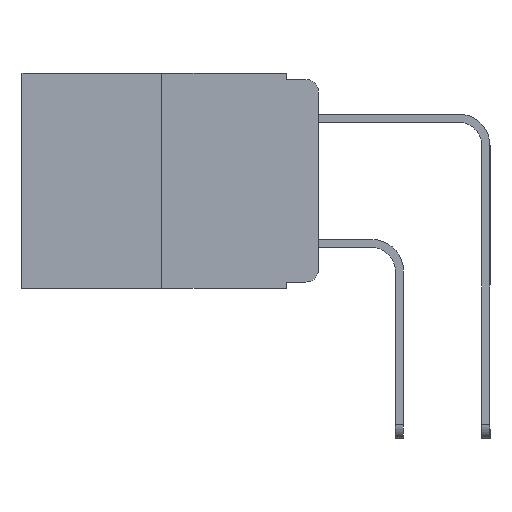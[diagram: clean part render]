
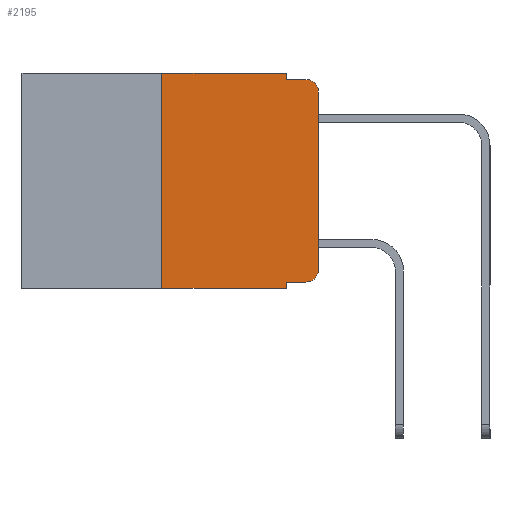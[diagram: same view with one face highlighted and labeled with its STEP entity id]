
A CAD part, left-side view. The second image highlights one B-rep face of the part: STEP entity #2195.
In plain terms, the highlighted planar face has unit normal (-1, 0, 0).
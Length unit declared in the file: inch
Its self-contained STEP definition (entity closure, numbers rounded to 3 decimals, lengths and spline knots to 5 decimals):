
#108 = CIRCLE ( 'NONE', #7573, 0.02 ) ;
#112 = LINE ( 'NONE', #2387, #3016 ) ;
#264 = PLANE ( 'NONE',  #1719 ) ;
#511 = ORIENTED_EDGE ( 'NONE', *, *, #7250, .F. ) ;
#671 = VERTEX_POINT ( 'NONE', #11287 ) ;
#692 = DIRECTION ( 'NONE',  ( 0., 0., -1. ) ) ;
#811 = CARTESIAN_POINT ( 'NONE',  ( 0., 0.473, 0. ) ) ;
#914 = ORIENTED_EDGE ( 'NONE', *, *, #9636, .T. ) ;
#960 = DIRECTION ( 'NONE',  ( 0., -1., 0. ) ) ;
#1039 = EDGE_CURVE ( 'NONE', #1323, #6311, #2866, .T. ) ;
#1323 = VERTEX_POINT ( 'NONE', #10983 ) ;
#1545 = ORIENTED_EDGE ( 'NONE', *, *, #4286, .T. ) ;
#1719 = AXIS2_PLACEMENT_3D ( 'NONE', #811, #10977, #692 ) ;
#1778 = EDGE_CURVE ( 'NONE', #13021, #4450, #8793, .T. ) ;
#1879 = ORIENTED_EDGE ( 'NONE', *, *, #8302, .F. ) ;
#2195 = ADVANCED_FACE ( 'NONE', ( #4832 ), #264, .F. ) ;
#2387 = CARTESIAN_POINT ( 'NONE',  ( 0., 0.051, -0.333 ) ) ;
#2488 = EDGE_CURVE ( 'NONE', #5828, #1323, #112, .T. ) ;
#2866 = CIRCLE ( 'NONE', #7673, 0.02 ) ;
#2902 = ORIENTED_EDGE ( 'NONE', *, *, #3530, .F. ) ;
#3016 = VECTOR ( 'NONE', #5678, 39.37008 ) ;
#3381 = VERTEX_POINT ( 'NONE', #6296 ) ;
#3505 = ORIENTED_EDGE ( 'NONE', *, *, #10499, .T. ) ;
#3530 = EDGE_CURVE ( 'NONE', #5439, #5777, #13121, .T. ) ;
#3542 = DIRECTION ( 'NONE',  ( 0., 0., -1. ) ) ;
#3568 = CARTESIAN_POINT ( 'NONE',  ( 0., 0.051, 0. ) ) ;
#3664 = LINE ( 'NONE', #7197, #8765 ) ;
#4161 = DIRECTION ( 'NONE',  ( 0., 0., 1. ) ) ;
#4286 = EDGE_CURVE ( 'NONE', #5439, #6856, #12035, .T. ) ;
#4387 = DIRECTION ( 'NONE',  ( 0., -1., 0. ) ) ;
#4450 = VERTEX_POINT ( 'NONE', #5473 ) ;
#4791 = CARTESIAN_POINT ( 'NONE',  ( 0., 0.02, -0.03 ) ) ;
#4832 = FACE_OUTER_BOUND ( 'NONE', #7672, .T. ) ;
#4852 = LINE ( 'NONE', #3568, #7277 ) ;
#4964 = CARTESIAN_POINT ( 'NONE',  ( 0., 0.25, 0. ) ) ;
#5337 = ORIENTED_EDGE ( 'NONE', *, *, #9364, .F. ) ;
#5439 = VERTEX_POINT ( 'NONE', #12141 ) ;
#5473 = CARTESIAN_POINT ( 'NONE',  ( 0., 0.051, -0.01 ) ) ;
#5671 = VECTOR ( 'NONE', #8072, 39.37008 ) ;
#5678 = DIRECTION ( 'NONE',  ( 0., -1., 0. ) ) ;
#5777 = VERTEX_POINT ( 'NONE', #8673 ) ;
#5828 = VERTEX_POINT ( 'NONE', #7780 ) ;
#5852 = DIRECTION ( 'NONE',  ( 0., 0., -1. ) ) ;
#6015 = LINE ( 'NONE', #7058, #5671 ) ;
#6269 = DIRECTION ( 'NONE',  ( -1., 0., 0. ) ) ;
#6296 = CARTESIAN_POINT ( 'NONE',  ( 0., 0., -0.03 ) ) ;
#6311 = VERTEX_POINT ( 'NONE', #8401 ) ;
#6856 = VERTEX_POINT ( 'NONE', #11225 ) ;
#7058 = CARTESIAN_POINT ( 'NONE',  ( 0., 0.051, -0.01 ) ) ;
#7197 = CARTESIAN_POINT ( 'NONE',  ( 0., 0., 0. ) ) ;
#7250 = EDGE_CURVE ( 'NONE', #4450, #671, #6015, .T. ) ;
#7277 = VECTOR ( 'NONE', #11674, 39.37008 ) ;
#7467 = CARTESIAN_POINT ( 'NONE',  ( 0., 0.473, 0. ) ) ;
#7573 = AXIS2_PLACEMENT_3D ( 'NONE', #4791, #11863, #5852 ) ;
#7672 = EDGE_LOOP ( 'NONE', ( #3505, #914, #511, #9010, #5337, #2902, #1545, #1879, #10424, #13045 ) ) ;
#7673 = AXIS2_PLACEMENT_3D ( 'NONE', #12060, #6269, #12127 ) ;
#7780 = CARTESIAN_POINT ( 'NONE',  ( 0., 0.051, -0.333 ) ) ;
#8072 = DIRECTION ( 'NONE',  ( 0., -1., 0. ) ) ;
#8115 = CARTESIAN_POINT ( 'NONE',  ( 0., 0.051, 0. ) ) ;
#8122 = DIRECTION ( 'NONE',  ( 0., 0., 1. ) ) ;
#8302 = EDGE_CURVE ( 'NONE', #5828, #6856, #4852, .T. ) ;
#8401 = CARTESIAN_POINT ( 'NONE',  ( 0., 0., -0.313 ) ) ;
#8673 = CARTESIAN_POINT ( 'NONE',  ( 0., 0.25, 0. ) ) ;
#8765 = VECTOR ( 'NONE', #4161, 39.37008 ) ;
#8793 = LINE ( 'NONE', #8115, #11016 ) ;
#9010 = ORIENTED_EDGE ( 'NONE', *, *, #1778, .F. ) ;
#9364 = EDGE_CURVE ( 'NONE', #5777, #13021, #13295, .T. ) ;
#9381 = VECTOR ( 'NONE', #960, 39.37008 ) ;
#9636 = EDGE_CURVE ( 'NONE', #3381, #671, #108, .T. ) ;
#10284 = CARTESIAN_POINT ( 'NONE',  ( 0., 0.051, 0. ) ) ;
#10424 = ORIENTED_EDGE ( 'NONE', *, *, #2488, .T. ) ;
#10499 = EDGE_CURVE ( 'NONE', #6311, #3381, #3664, .T. ) ;
#10697 = VECTOR ( 'NONE', #4387, 39.37008 ) ;
#10977 = DIRECTION ( 'NONE',  ( 1., 0., 0. ) ) ;
#10983 = CARTESIAN_POINT ( 'NONE',  ( 0., 0.02, -0.333 ) ) ;
#11016 = VECTOR ( 'NONE', #3542, 39.37008 ) ;
#11225 = CARTESIAN_POINT ( 'NONE',  ( 0., 0.051, -0.343 ) ) ;
#11287 = CARTESIAN_POINT ( 'NONE',  ( 0., 0.02, -0.01 ) ) ;
#11674 = DIRECTION ( 'NONE',  ( 0., 0., -1. ) ) ;
#11863 = DIRECTION ( 'NONE',  ( -1., 0., 0. ) ) ;
#12035 = LINE ( 'NONE', #12240, #9381 ) ;
#12060 = CARTESIAN_POINT ( 'NONE',  ( 0., 0.02, -0.313 ) ) ;
#12127 = DIRECTION ( 'NONE',  ( 0., 0., -1. ) ) ;
#12141 = CARTESIAN_POINT ( 'NONE',  ( 0., 0.25, -0.343 ) ) ;
#12240 = CARTESIAN_POINT ( 'NONE',  ( 0., 0.473, -0.343 ) ) ;
#12817 = VECTOR ( 'NONE', #8122, 39.37008 ) ;
#13021 = VERTEX_POINT ( 'NONE', #10284 ) ;
#13045 = ORIENTED_EDGE ( 'NONE', *, *, #1039, .T. ) ;
#13121 = LINE ( 'NONE', #4964, #12817 ) ;
#13295 = LINE ( 'NONE', #7467, #10697 ) ;
